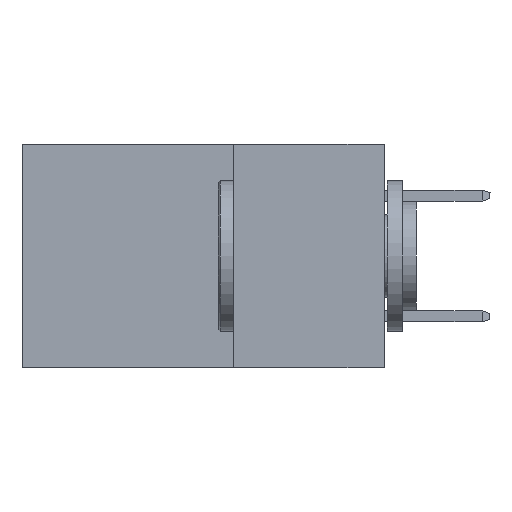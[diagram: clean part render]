
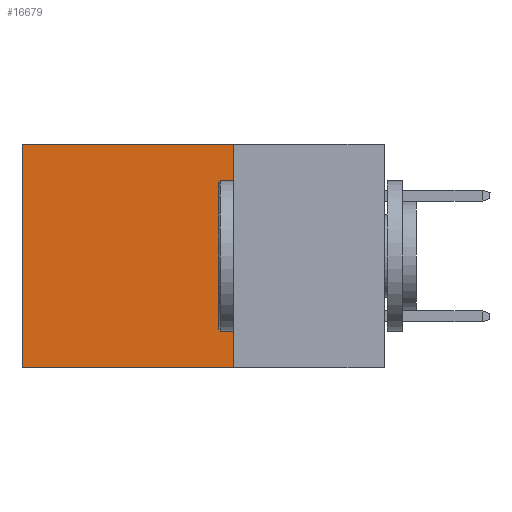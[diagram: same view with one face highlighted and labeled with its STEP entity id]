
A CAD part, left-side view. The second image highlights one B-rep face of the part: STEP entity #16679.
In plain terms, the highlighted planar face has unit normal (-1, 0, 0).
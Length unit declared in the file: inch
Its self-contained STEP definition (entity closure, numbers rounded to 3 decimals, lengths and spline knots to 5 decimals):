
#861 = LINE ( 'NONE', #11937, #7064 ) ;
#1091 = VERTEX_POINT ( 'NONE', #8700 ) ;
#1316 = VECTOR ( 'NONE', #5230, 39.37008 ) ;
#1670 = CARTESIAN_POINT ( 'NONE',  ( 0.298, 0.6, 0. ) ) ;
#1696 = ORIENTED_EDGE ( 'NONE', *, *, #10994, .T. ) ;
#2055 = CARTESIAN_POINT ( 'NONE',  ( 0.298, 0.25, 0. ) ) ;
#2308 = CARTESIAN_POINT ( 'NONE',  ( 0.298, 0.25, 0. ) ) ;
#2610 = CARTESIAN_POINT ( 'NONE',  ( 0.298, 0.25, -0.37 ) ) ;
#2993 = EDGE_CURVE ( 'NONE', #17727, #12332, #14401, .T. ) ;
#3802 = FACE_OUTER_BOUND ( 'NONE', #13248, .T. ) ;
#4563 = VERTEX_POINT ( 'NONE', #1670 ) ;
#4921 = PLANE ( 'NONE',  #10204 ) ;
#5083 = CARTESIAN_POINT ( 'NONE',  ( 0.298, 0.25, -0.37 ) ) ;
#5230 = DIRECTION ( 'NONE',  ( 0., 1., 0. ) ) ;
#6595 = CARTESIAN_POINT ( 'NONE',  ( 0.298, 0.6, 0. ) ) ;
#7064 = VECTOR ( 'NONE', #14741, 39.37008 ) ;
#7097 = LINE ( 'NONE', #2610, #1316 ) ;
#8346 = CARTESIAN_POINT ( 'NONE',  ( 0.298, 0.25, 0. ) ) ;
#8700 = CARTESIAN_POINT ( 'NONE',  ( 0.298, 0.6, -0.37 ) ) ;
#8746 = VECTOR ( 'NONE', #9296, 39.37008 ) ;
#8986 = ORIENTED_EDGE ( 'NONE', *, *, #14137, .F. ) ;
#9178 = DIRECTION ( 'NONE',  ( 1., 0., 0. ) ) ;
#9296 = DIRECTION ( 'NONE',  ( 0., 0., -1. ) ) ;
#10204 = AXIS2_PLACEMENT_3D ( 'NONE', #2308, #9178, #11953 ) ;
#10994 = EDGE_CURVE ( 'NONE', #17727, #4563, #861, .T. ) ;
#11790 = EDGE_CURVE ( 'NONE', #4563, #1091, #14600, .T. ) ;
#11937 = CARTESIAN_POINT ( 'NONE',  ( 0.298, 0.25, 0. ) ) ;
#11953 = DIRECTION ( 'NONE',  ( 0., 0., -1. ) ) ;
#12332 = VERTEX_POINT ( 'NONE', #5083 ) ;
#12876 = VECTOR ( 'NONE', #16596, 39.37008 ) ;
#13248 = EDGE_LOOP ( 'NONE', ( #14763, #8986, #16099, #1696 ) ) ;
#14137 = EDGE_CURVE ( 'NONE', #12332, #1091, #7097, .T. ) ;
#14401 = LINE ( 'NONE', #8346, #12876 ) ;
#14600 = LINE ( 'NONE', #6595, #8746 ) ;
#14741 = DIRECTION ( 'NONE',  ( 0., 1., 0. ) ) ;
#14763 = ORIENTED_EDGE ( 'NONE', *, *, #11790, .T. ) ;
#16099 = ORIENTED_EDGE ( 'NONE', *, *, #2993, .F. ) ;
#16596 = DIRECTION ( 'NONE',  ( 0., 0., -1. ) ) ;
#16679 = ADVANCED_FACE ( 'NONE', ( #3802 ), #4921, .F. ) ;
#17727 = VERTEX_POINT ( 'NONE', #2055 ) ;
